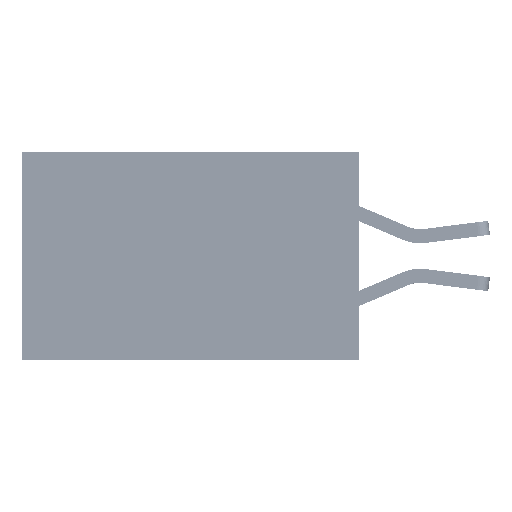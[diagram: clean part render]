
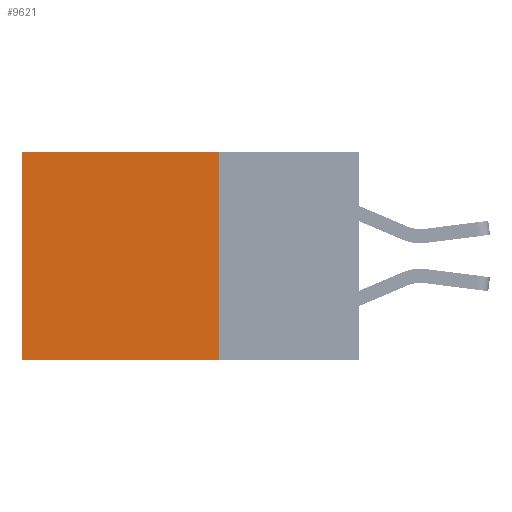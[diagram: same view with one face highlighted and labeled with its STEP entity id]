
A CAD part, left-side view. The second image highlights one B-rep face of the part: STEP entity #9621.
In plain terms, the highlighted planar face has unit normal (-1, 0, 0).
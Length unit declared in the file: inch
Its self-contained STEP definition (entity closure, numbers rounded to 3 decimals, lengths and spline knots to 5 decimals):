
#2490 = CARTESIAN_POINT ( 'NONE',  ( 0.2875, 0.6, -0.37 ) ) ;
#3719 = VERTEX_POINT ( 'NONE', #2490 ) ;
#5373 = VECTOR ( 'NONE', #43138, 39.37008 ) ;
#8644 = DIRECTION ( 'NONE',  ( 0., 0., -1. ) ) ;
#8681 = VERTEX_POINT ( 'NONE', #15199 ) ;
#9621 = ADVANCED_FACE ( 'NONE', ( #27366 ), #15650, .F. ) ;
#10877 = EDGE_CURVE ( 'NONE', #8681, #15025, #39617, .T. ) ;
#12104 = CARTESIAN_POINT ( 'NONE',  ( 0.2875, 0.25, 0. ) ) ;
#12141 = CARTESIAN_POINT ( 'NONE',  ( 0.2875, 0.25, -0.37 ) ) ;
#12296 = VECTOR ( 'NONE', #8644, 39.37008 ) ;
#14988 = VECTOR ( 'NONE', #32466, 39.37008 ) ;
#15025 = VERTEX_POINT ( 'NONE', #12141 ) ;
#15199 = CARTESIAN_POINT ( 'NONE',  ( 0.2875, 0.25, 0. ) ) ;
#15650 = PLANE ( 'NONE',  #25689 ) ;
#15731 = ORIENTED_EDGE ( 'NONE', *, *, #25847, .F. ) ;
#19732 = CARTESIAN_POINT ( 'NONE',  ( 0.2875, 0.6, 0. ) ) ;
#21681 = EDGE_LOOP ( 'NONE', ( #32954, #15731, #35237, #43200 ) ) ;
#22122 = CARTESIAN_POINT ( 'NONE',  ( 0.2875, 0.25, -0.37 ) ) ;
#22593 = CARTESIAN_POINT ( 'NONE',  ( 0.2875, 0.6, 0. ) ) ;
#22672 = DIRECTION ( 'NONE',  ( 0., 0., -1. ) ) ;
#25689 = AXIS2_PLACEMENT_3D ( 'NONE', #36322, #43224, #22672 ) ;
#25847 = EDGE_CURVE ( 'NONE', #15025, #3719, #34330, .T. ) ;
#27366 = FACE_OUTER_BOUND ( 'NONE', #21681, .T. ) ;
#32466 = DIRECTION ( 'NONE',  ( 0., 1., 0. ) ) ;
#32954 = ORIENTED_EDGE ( 'NONE', *, *, #41526, .T. ) ;
#32966 = EDGE_CURVE ( 'NONE', #8681, #34386, #41823, .T. ) ;
#34330 = LINE ( 'NONE', #22122, #14988 ) ;
#34386 = VERTEX_POINT ( 'NONE', #22593 ) ;
#35237 = ORIENTED_EDGE ( 'NONE', *, *, #10877, .F. ) ;
#36322 = CARTESIAN_POINT ( 'NONE',  ( 0.2875, 0.25, 0. ) ) ;
#37894 = VECTOR ( 'NONE', #40281, 39.37008 ) ;
#39617 = LINE ( 'NONE', #12104, #12296 ) ;
#39662 = CARTESIAN_POINT ( 'NONE',  ( 0.2875, 0.25, 0. ) ) ;
#40063 = LINE ( 'NONE', #19732, #37894 ) ;
#40281 = DIRECTION ( 'NONE',  ( 0., 0., -1. ) ) ;
#41526 = EDGE_CURVE ( 'NONE', #34386, #3719, #40063, .T. ) ;
#41823 = LINE ( 'NONE', #39662, #5373 ) ;
#43138 = DIRECTION ( 'NONE',  ( 0., 1., 0. ) ) ;
#43200 = ORIENTED_EDGE ( 'NONE', *, *, #32966, .T. ) ;
#43224 = DIRECTION ( 'NONE',  ( 1., 0., 0. ) ) ;
